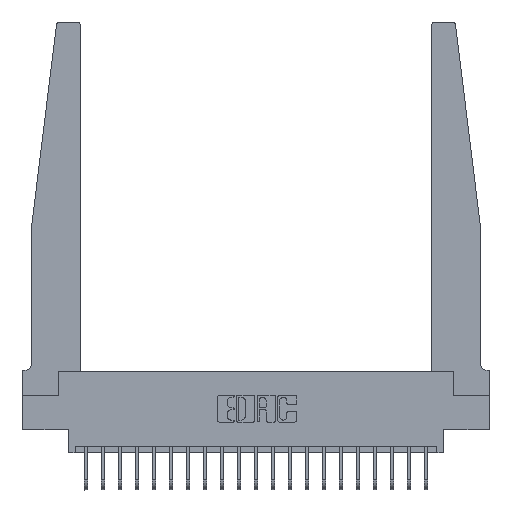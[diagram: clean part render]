
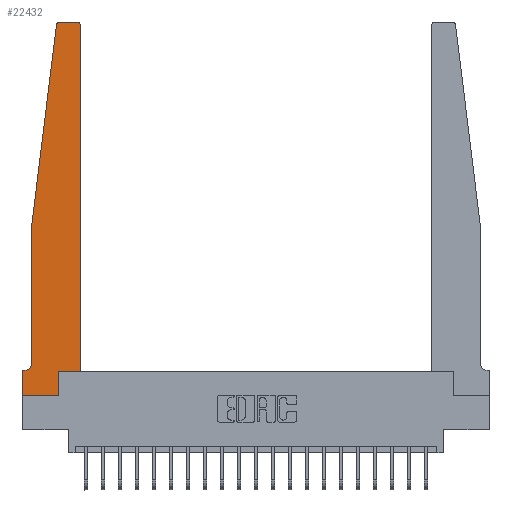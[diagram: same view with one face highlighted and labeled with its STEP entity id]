
A CAD part, top view. The second image highlights one B-rep face of the part: STEP entity #22432.
In plain terms, the highlighted planar face has unit normal (0, 0, 1).
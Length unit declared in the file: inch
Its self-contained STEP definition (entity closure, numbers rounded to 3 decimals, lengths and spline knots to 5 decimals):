
#143 = DIRECTION ( 'NONE',  ( 0., -1., 0. ) ) ;
#158 = CIRCLE ( 'NONE', #10984, 0.03 ) ;
#175 = AXIS2_PLACEMENT_3D ( 'NONE', #4274, #4358, #9680 ) ;
#252 = DIRECTION ( 'NONE',  ( 1., 0., 0. ) ) ;
#419 = CARTESIAN_POINT ( 'NONE',  ( 0.065, 1.25, 0.37 ) ) ;
#496 = EDGE_CURVE ( 'NONE', #16411, #1397, #158, .T. ) ;
#528 = LINE ( 'NONE', #7354, #1924 ) ;
#575 = AXIS2_PLACEMENT_3D ( 'NONE', #16459, #14744, #11143 ) ;
#1397 = VERTEX_POINT ( 'NONE', #14457 ) ;
#1488 = CARTESIAN_POINT ( 'NONE',  ( 0.27653, 2.72, 0.37 ) ) ;
#1863 = VERTEX_POINT ( 'NONE', #15615 ) ;
#1924 = VECTOR ( 'NONE', #252, 39.37008 ) ;
#2202 = CARTESIAN_POINT ( 'NONE',  ( 0.25, 2.75, 0.37 ) ) ;
#2685 = CARTESIAN_POINT ( 'NONE',  ( 0.425, 0.18, 0.37 ) ) ;
#2719 = DIRECTION ( 'NONE',  ( 1., 0., 0. ) ) ;
#2891 = ORIENTED_EDGE ( 'NONE', *, *, #21594, .T. ) ;
#2952 = CARTESIAN_POINT ( 'NONE',  ( 0., 0., 0.37 ) ) ;
#3137 = EDGE_CURVE ( 'NONE', #3440, #1863, #8539, .T. ) ;
#3332 = VECTOR ( 'NONE', #10933, 39.37008 ) ;
#3428 = ORIENTED_EDGE ( 'NONE', *, *, #4211, .T. ) ;
#3440 = VERTEX_POINT ( 'NONE', #10021 ) ;
#3520 = EDGE_CURVE ( 'NONE', #22463, #11154, #20012, .T. ) ;
#3599 = VERTEX_POINT ( 'NONE', #2685 ) ;
#3882 = LINE ( 'NONE', #7151, #3332 ) ;
#4211 = EDGE_CURVE ( 'NONE', #11878, #5322, #9877, .T. ) ;
#4274 = CARTESIAN_POINT ( 'NONE',  ( 0., 0.1875, 0.37 ) ) ;
#4358 = DIRECTION ( 'NONE',  ( 0., 0., 1. ) ) ;
#4727 = VECTOR ( 'NONE', #7938, 39.37008 ) ;
#5305 = LINE ( 'NONE', #15334, #4727 ) ;
#5322 = VERTEX_POINT ( 'NONE', #15614 ) ;
#5515 = CARTESIAN_POINT ( 'NONE',  ( 0.065, 1.25, 0.37 ) ) ;
#6065 = DIRECTION ( 'NONE',  ( 0., 0., 1. ) ) ;
#6122 = CARTESIAN_POINT ( 'NONE',  ( 0.27653, 2.75, 0.37 ) ) ;
#6534 = CIRCLE ( 'NONE', #22339, 0.03 ) ;
#7059 = DIRECTION ( 'NONE',  ( 0., 1., 0. ) ) ;
#7151 = CARTESIAN_POINT ( 'NONE',  ( 0.065, 1.25, 0.37 ) ) ;
#7354 = CARTESIAN_POINT ( 'NONE',  ( 0.425, 0.18, 0.37 ) ) ;
#7370 = DIRECTION ( 'NONE',  ( 0., 1., 0. ) ) ;
#7508 = VERTEX_POINT ( 'NONE', #18108 ) ;
#7856 = VECTOR ( 'NONE', #11145, 39.37008 ) ;
#7907 = EDGE_CURVE ( 'NONE', #14249, #7508, #6534, .T. ) ;
#7938 = DIRECTION ( 'NONE',  ( -1., 0., 0. ) ) ;
#8114 = FACE_OUTER_BOUND ( 'NONE', #14361, .T. ) ;
#8539 = LINE ( 'NONE', #19899, #13039 ) ;
#9203 = LINE ( 'NONE', #5515, #17607 ) ;
#9680 = DIRECTION ( 'NONE',  ( 1., 0., 0. ) ) ;
#9877 = CIRCLE ( 'NONE', #575, 0.05 ) ;
#9903 = VERTEX_POINT ( 'NONE', #419 ) ;
#10021 = CARTESIAN_POINT ( 'NONE',  ( 0.2605, 0., 0.37 ) ) ;
#10111 = LINE ( 'NONE', #10570, #19931 ) ;
#10279 = EDGE_CURVE ( 'NONE', #11154, #3440, #10111, .T. ) ;
#10570 = CARTESIAN_POINT ( 'NONE',  ( 0., 0., 0.37 ) ) ;
#10933 = DIRECTION ( 'NONE',  ( -0.122, -0.992, 0. ) ) ;
#10984 = AXIS2_PLACEMENT_3D ( 'NONE', #13463, #6065, #2719 ) ;
#11143 = DIRECTION ( 'NONE',  ( -1., 0., 0. ) ) ;
#11145 = DIRECTION ( 'NONE',  ( -1., 0., 0. ) ) ;
#11154 = VERTEX_POINT ( 'NONE', #2952 ) ;
#11534 = CARTESIAN_POINT ( 'NONE',  ( 0., 0., 0.37 ) ) ;
#11878 = VERTEX_POINT ( 'NONE', #17259 ) ;
#12215 = ORIENTED_EDGE ( 'NONE', *, *, #12934, .T. ) ;
#12928 = LINE ( 'NONE', #2202, #7856 ) ;
#12934 = EDGE_CURVE ( 'NONE', #3599, #16411, #18356, .T. ) ;
#13039 = VECTOR ( 'NONE', #7059, 39.37008 ) ;
#13352 = DIRECTION ( 'NONE',  ( 0., -1., 0. ) ) ;
#13463 = CARTESIAN_POINT ( 'NONE',  ( 0.395, 2.72, 0.37 ) ) ;
#14249 = VERTEX_POINT ( 'NONE', #6122 ) ;
#14361 = EDGE_LOOP ( 'NONE', ( #16472, #18157, #14877, #17176, #3428, #14960, #15280, #19605, #16881, #2891, #12215, #22853 ) ) ;
#14446 = CARTESIAN_POINT ( 'NONE',  ( 0.425, 2.72, 0.37 ) ) ;
#14457 = CARTESIAN_POINT ( 'NONE',  ( 0.395, 2.75, 0.37 ) ) ;
#14744 = DIRECTION ( 'NONE',  ( 0., 0., -1. ) ) ;
#14877 = ORIENTED_EDGE ( 'NONE', *, *, #20716, .T. ) ;
#14960 = ORIENTED_EDGE ( 'NONE', *, *, #22466, .T. ) ;
#15176 = PLANE ( 'NONE',  #175 ) ;
#15280 = ORIENTED_EDGE ( 'NONE', *, *, #3520, .T. ) ;
#15334 = CARTESIAN_POINT ( 'NONE',  ( 0.065, 0.1875, 0.37 ) ) ;
#15614 = CARTESIAN_POINT ( 'NONE',  ( 0.015, 0.1875, 0.37 ) ) ;
#15615 = CARTESIAN_POINT ( 'NONE',  ( 0.2605, 0.18, 0.37 ) ) ;
#16411 = VERTEX_POINT ( 'NONE', #14446 ) ;
#16459 = CARTESIAN_POINT ( 'NONE',  ( 0.015, 0.2375, 0.37 ) ) ;
#16472 = ORIENTED_EDGE ( 'NONE', *, *, #21560, .T. ) ;
#16881 = ORIENTED_EDGE ( 'NONE', *, *, #3137, .T. ) ;
#16967 = VECTOR ( 'NONE', #7370, 39.37008 ) ;
#17176 = ORIENTED_EDGE ( 'NONE', *, *, #18000, .T. ) ;
#17259 = CARTESIAN_POINT ( 'NONE',  ( 0.065, 0.2375, 0.37 ) ) ;
#17607 = VECTOR ( 'NONE', #143, 39.37008 ) ;
#17678 = DIRECTION ( 'NONE',  ( 1., 0., 0. ) ) ;
#17845 = DIRECTION ( 'NONE',  ( 0., 0., 1. ) ) ;
#18000 = EDGE_CURVE ( 'NONE', #9903, #11878, #9203, .T. ) ;
#18108 = CARTESIAN_POINT ( 'NONE',  ( 0.24675, 2.72367, 0.37 ) ) ;
#18157 = ORIENTED_EDGE ( 'NONE', *, *, #7907, .T. ) ;
#18356 = LINE ( 'NONE', #19992, #16967 ) ;
#19605 = ORIENTED_EDGE ( 'NONE', *, *, #10279, .T. ) ;
#19729 = VECTOR ( 'NONE', #13352, 39.37008 ) ;
#19899 = CARTESIAN_POINT ( 'NONE',  ( 0.2605, 0.18, 0.37 ) ) ;
#19931 = VECTOR ( 'NONE', #23060, 39.37008 ) ;
#19992 = CARTESIAN_POINT ( 'NONE',  ( 0.425, 0.18, 0.37 ) ) ;
#20012 = LINE ( 'NONE', #11534, #19729 ) ;
#20541 = CARTESIAN_POINT ( 'NONE',  ( 0., 0.1875, 0.37 ) ) ;
#20716 = EDGE_CURVE ( 'NONE', #7508, #9903, #3882, .T. ) ;
#21560 = EDGE_CURVE ( 'NONE', #1397, #14249, #12928, .T. ) ;
#21594 = EDGE_CURVE ( 'NONE', #1863, #3599, #528, .T. ) ;
#22339 = AXIS2_PLACEMENT_3D ( 'NONE', #1488, #17845, #17678 ) ;
#22432 = ADVANCED_FACE ( 'NONE', ( #8114 ), #15176, .T. ) ;
#22463 = VERTEX_POINT ( 'NONE', #20541 ) ;
#22466 = EDGE_CURVE ( 'NONE', #5322, #22463, #5305, .T. ) ;
#22853 = ORIENTED_EDGE ( 'NONE', *, *, #496, .T. ) ;
#23060 = DIRECTION ( 'NONE',  ( 1., 0., 0. ) ) ;
